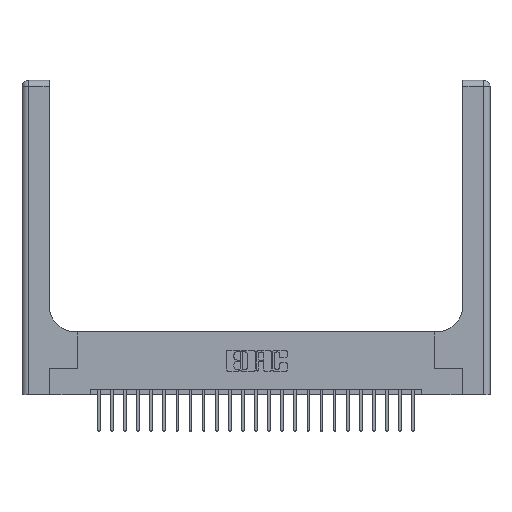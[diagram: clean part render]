
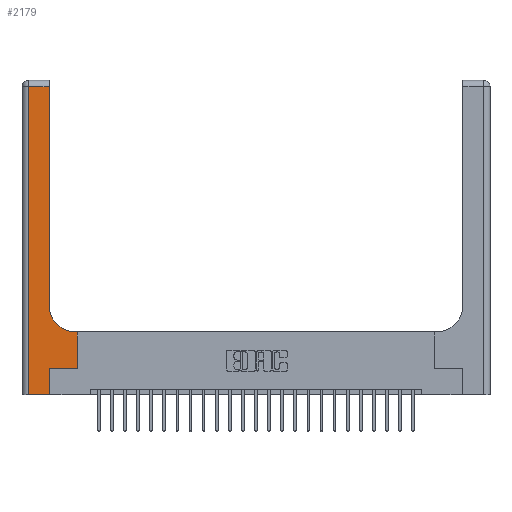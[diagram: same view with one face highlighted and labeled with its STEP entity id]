
A CAD part, top view. The second image highlights one B-rep face of the part: STEP entity #2179.
In plain terms, the highlighted planar face has unit normal (0, 0, 1).
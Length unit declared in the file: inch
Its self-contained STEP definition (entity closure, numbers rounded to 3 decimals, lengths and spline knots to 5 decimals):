
#276 = DIRECTION ( 'NONE',  ( 1., 0., 0. ) ) ;
#1021 = DIRECTION ( 'NONE',  ( 1., 0., 0. ) ) ;
#1027 = AXIS2_PLACEMENT_3D ( 'NONE', #21838, #21467, #17783 ) ;
#1170 = DIRECTION ( 'NONE',  ( 0., 1., 0. ) ) ;
#1706 = ORIENTED_EDGE ( 'NONE', *, *, #2533, .T. ) ;
#1861 = ORIENTED_EDGE ( 'NONE', *, *, #13589, .T. ) ;
#1997 = ORIENTED_EDGE ( 'NONE', *, *, #10798, .T. ) ;
#2108 = LINE ( 'NONE', #6030, #10101 ) ;
#2179 = ADVANCED_FACE ( 'NONE', ( #12254 ), #19619, .F. ) ;
#2348 = LINE ( 'NONE', #9972, #5916 ) ;
#2488 = EDGE_CURVE ( 'NONE', #4481, #22077, #19717, .T. ) ;
#2533 = EDGE_CURVE ( 'NONE', #24181, #17931, #19846, .T. ) ;
#2808 = EDGE_CURVE ( 'NONE', #17620, #24181, #7792, .T. ) ;
#2851 = LINE ( 'NONE', #23491, #7948 ) ;
#3116 = DIRECTION ( 'NONE',  ( -1., 0., 0. ) ) ;
#3557 = ORIENTED_EDGE ( 'NONE', *, *, #7024, .T. ) ;
#3576 = CARTESIAN_POINT ( 'NONE',  ( 0.06, 2.94, 0.37 ) ) ;
#3980 = VECTOR ( 'NONE', #23954, 39.37008 ) ;
#4279 = ORIENTED_EDGE ( 'NONE', *, *, #2488, .T. ) ;
#4481 = VERTEX_POINT ( 'NONE', #3576 ) ;
#4573 = VECTOR ( 'NONE', #20797, 39.37008 ) ;
#4943 = CIRCLE ( 'NONE', #12018, 0.25 ) ;
#4987 = ORIENTED_EDGE ( 'NONE', *, *, #10453, .T. ) ;
#5916 = VECTOR ( 'NONE', #21150, 39.37008 ) ;
#5961 = CARTESIAN_POINT ( 'NONE',  ( 0.265, 0.25, 0.37 ) ) ;
#6030 = CARTESIAN_POINT ( 'NONE',  ( 0.265, 0.25, 0.37 ) ) ;
#6439 = CARTESIAN_POINT ( 'NONE',  ( 0.06, 3., 0.37 ) ) ;
#6513 = VECTOR ( 'NONE', #13946, 39.37008 ) ;
#6894 = DIRECTION ( 'NONE',  ( 0., 0., -1. ) ) ;
#7024 = EDGE_CURVE ( 'NONE', #21279, #17620, #2108, .T. ) ;
#7621 = CARTESIAN_POINT ( 'NONE',  ( 0.26, 0.85, 0.37 ) ) ;
#7629 = EDGE_CURVE ( 'NONE', #8777, #21279, #23410, .T. ) ;
#7792 = LINE ( 'NONE', #13568, #4573 ) ;
#7940 = ORIENTED_EDGE ( 'NONE', *, *, #20186, .T. ) ;
#7948 = VECTOR ( 'NONE', #1021, 39.37008 ) ;
#8597 = VERTEX_POINT ( 'NONE', #12298 ) ;
#8664 = CARTESIAN_POINT ( 'NONE',  ( 0.265, 0., 0.37 ) ) ;
#8777 = VERTEX_POINT ( 'NONE', #18183 ) ;
#9896 = ORIENTED_EDGE ( 'NONE', *, *, #7629, .T. ) ;
#9972 = CARTESIAN_POINT ( 'NONE',  ( 0., 2.94, 0.37 ) ) ;
#10101 = VECTOR ( 'NONE', #276, 39.37008 ) ;
#10453 = EDGE_CURVE ( 'NONE', #8597, #4481, #2348, .T. ) ;
#10798 = EDGE_CURVE ( 'NONE', #23726, #8597, #14974, .T. ) ;
#11261 = CARTESIAN_POINT ( 'NONE',  ( 0.51, 0.6, 0.37 ) ) ;
#12018 = AXIS2_PLACEMENT_3D ( 'NONE', #14744, #6894, #21890 ) ;
#12254 = FACE_OUTER_BOUND ( 'NONE', #12757, .T. ) ;
#12298 = CARTESIAN_POINT ( 'NONE',  ( 0.26, 2.94, 0.37 ) ) ;
#12757 = EDGE_LOOP ( 'NONE', ( #1997, #4987, #4279, #1861, #9896, #3557, #20367, #1706, #7940 ) ) ;
#13568 = CARTESIAN_POINT ( 'NONE',  ( 0.528, 0.25, 0.37 ) ) ;
#13589 = EDGE_CURVE ( 'NONE', #22077, #8777, #2851, .T. ) ;
#13946 = DIRECTION ( 'NONE',  ( 0., -1., 0. ) ) ;
#14744 = CARTESIAN_POINT ( 'NONE',  ( 0.51, 0.85, 0.37 ) ) ;
#14873 = CARTESIAN_POINT ( 'NONE',  ( 0.06, 0., 0.37 ) ) ;
#14974 = LINE ( 'NONE', #18555, #3980 ) ;
#17075 = CARTESIAN_POINT ( 'NONE',  ( 0.528, 0.25, 0.37 ) ) ;
#17620 = VERTEX_POINT ( 'NONE', #17075 ) ;
#17783 = DIRECTION ( 'NONE',  ( -1., 0., 0. ) ) ;
#17931 = VERTEX_POINT ( 'NONE', #11261 ) ;
#17987 = CARTESIAN_POINT ( 'NONE',  ( 0.26, 0.6, 0.37 ) ) ;
#18183 = CARTESIAN_POINT ( 'NONE',  ( 0.265, 0., 0.37 ) ) ;
#18555 = CARTESIAN_POINT ( 'NONE',  ( 0.26, 3., 0.37 ) ) ;
#19619 = PLANE ( 'NONE',  #1027 ) ;
#19717 = LINE ( 'NONE', #6439, #6513 ) ;
#19846 = LINE ( 'NONE', #17987, #20655 ) ;
#20186 = EDGE_CURVE ( 'NONE', #17931, #23726, #4943, .T. ) ;
#20367 = ORIENTED_EDGE ( 'NONE', *, *, #2808, .T. ) ;
#20482 = CARTESIAN_POINT ( 'NONE',  ( 0.528, 0.6, 0.37 ) ) ;
#20655 = VECTOR ( 'NONE', #3116, 39.37008 ) ;
#20797 = DIRECTION ( 'NONE',  ( 0., 1., 0. ) ) ;
#21150 = DIRECTION ( 'NONE',  ( -1., 0., 0. ) ) ;
#21279 = VERTEX_POINT ( 'NONE', #5961 ) ;
#21467 = DIRECTION ( 'NONE',  ( 0., 0., -1. ) ) ;
#21838 = CARTESIAN_POINT ( 'NONE',  ( 0., 3., 0.37 ) ) ;
#21890 = DIRECTION ( 'NONE',  ( 1., 0., 0. ) ) ;
#22077 = VERTEX_POINT ( 'NONE', #14873 ) ;
#23319 = VECTOR ( 'NONE', #1170, 39.37008 ) ;
#23410 = LINE ( 'NONE', #8664, #23319 ) ;
#23491 = CARTESIAN_POINT ( 'NONE',  ( 0., 0., 0.37 ) ) ;
#23726 = VERTEX_POINT ( 'NONE', #7621 ) ;
#23954 = DIRECTION ( 'NONE',  ( 0., 1., 0. ) ) ;
#24181 = VERTEX_POINT ( 'NONE', #20482 ) ;
